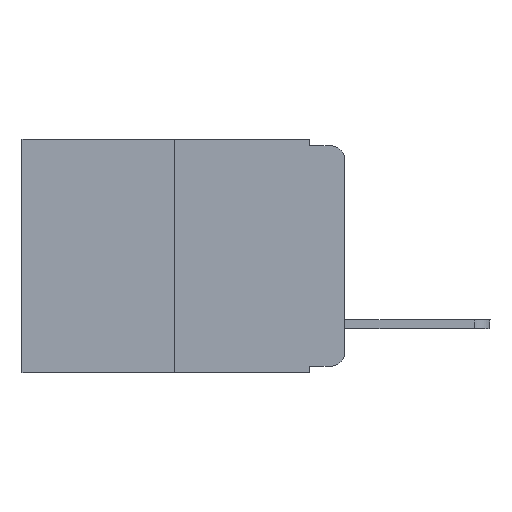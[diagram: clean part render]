
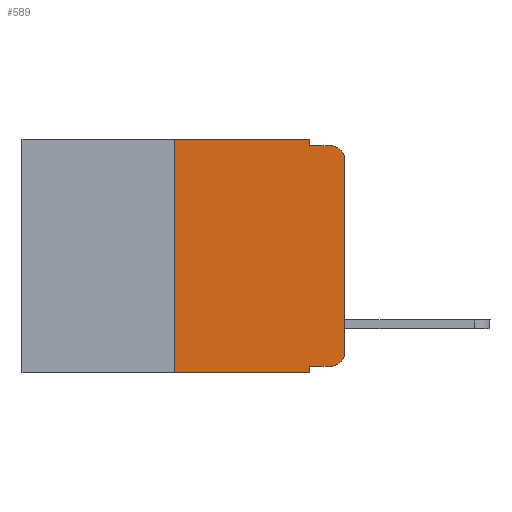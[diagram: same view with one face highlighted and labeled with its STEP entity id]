
A CAD part, left-side view. The second image highlights one B-rep face of the part: STEP entity #589.
In plain terms, the highlighted planar face has unit normal (-1, 0, 0).
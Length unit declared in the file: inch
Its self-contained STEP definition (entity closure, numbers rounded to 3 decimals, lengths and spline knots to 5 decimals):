
#64 = DIRECTION ( 'NONE',  ( 0., -1., 0. ) ) ;
#264 = EDGE_CURVE ( 'NONE', #17933, #17940, #12349, .T. ) ;
#484 = AXIS2_PLACEMENT_3D ( 'NONE', #14368, #19303, #11147 ) ;
#589 = ADVANCED_FACE ( 'NONE', ( #12611 ), #6044, .F. ) ;
#773 = ORIENTED_EDGE ( 'NONE', *, *, #10100, .T. ) ;
#1182 = CARTESIAN_POINT ( 'NONE',  ( 0., 0.051, 0. ) ) ;
#1595 = DIRECTION ( 'NONE',  ( 0., 0., 1. ) ) ;
#1797 = ORIENTED_EDGE ( 'NONE', *, *, #4053, .F. ) ;
#2514 = VERTEX_POINT ( 'NONE', #8550 ) ;
#2700 = CARTESIAN_POINT ( 'NONE',  ( 0., 0., -0.03 ) ) ;
#2999 = CARTESIAN_POINT ( 'NONE',  ( 0., 0., 0. ) ) ;
#3003 = VECTOR ( 'NONE', #1595, 39.37008 ) ;
#3237 = DIRECTION ( 'NONE',  ( 0., 0., -1. ) ) ;
#3683 = ORIENTED_EDGE ( 'NONE', *, *, #20851, .T. ) ;
#3933 = CARTESIAN_POINT ( 'NONE',  ( 0., 0.051, -0.01 ) ) ;
#4053 = EDGE_CURVE ( 'NONE', #6604, #7138, #17782, .T. ) ;
#4544 = CARTESIAN_POINT ( 'NONE',  ( 0., 0.051, 0. ) ) ;
#4572 = CARTESIAN_POINT ( 'NONE',  ( 0., 0.051, -0.333 ) ) ;
#4611 = ORIENTED_EDGE ( 'NONE', *, *, #19996, .F. ) ;
#4743 = ORIENTED_EDGE ( 'NONE', *, *, #8467, .F. ) ;
#4758 = CARTESIAN_POINT ( 'NONE',  ( 0., 0.02, -0.01 ) ) ;
#5147 = ORIENTED_EDGE ( 'NONE', *, *, #264, .T. ) ;
#6044 = PLANE ( 'NONE',  #15640 ) ;
#6058 = DIRECTION ( 'NONE',  ( 0., 0., -1. ) ) ;
#6085 = LINE ( 'NONE', #4572, #15547 ) ;
#6604 = VERTEX_POINT ( 'NONE', #19580 ) ;
#6805 = DIRECTION ( 'NONE',  ( -1., 0., 0. ) ) ;
#7040 = CIRCLE ( 'NONE', #484, 0.02 ) ;
#7138 = VERTEX_POINT ( 'NONE', #3933 ) ;
#7621 = CARTESIAN_POINT ( 'NONE',  ( 0., 0.02, -0.333 ) ) ;
#7890 = CARTESIAN_POINT ( 'NONE',  ( 0., 0.051, -0.01 ) ) ;
#8227 = VERTEX_POINT ( 'NONE', #18062 ) ;
#8467 = EDGE_CURVE ( 'NONE', #8227, #13539, #11939, .T. ) ;
#8550 = CARTESIAN_POINT ( 'NONE',  ( 0., 0., -0.313 ) ) ;
#9002 = ORIENTED_EDGE ( 'NONE', *, *, #15428, .T. ) ;
#9029 = CARTESIAN_POINT ( 'NONE',  ( 0., 0.25, 0. ) ) ;
#9471 = VECTOR ( 'NONE', #12783, 39.37008 ) ;
#9500 = CARTESIAN_POINT ( 'NONE',  ( 0., 0.473, 0. ) ) ;
#9531 = EDGE_CURVE ( 'NONE', #7138, #17940, #14756, .T. ) ;
#9762 = DIRECTION ( 'NONE',  ( 0., -1., 0. ) ) ;
#10100 = EDGE_CURVE ( 'NONE', #15686, #2514, #7040, .T. ) ;
#10711 = VECTOR ( 'NONE', #64, 39.37008 ) ;
#10806 = LINE ( 'NONE', #4544, #18174 ) ;
#11015 = DIRECTION ( 'NONE',  ( 0., -1., 0. ) ) ;
#11147 = DIRECTION ( 'NONE',  ( 0., 0., -1. ) ) ;
#11233 = VECTOR ( 'NONE', #11015, 39.37008 ) ;
#11670 = EDGE_CURVE ( 'NONE', #8227, #17687, #14346, .T. ) ;
#11675 = AXIS2_PLACEMENT_3D ( 'NONE', #14669, #6805, #3237 ) ;
#11805 = ORIENTED_EDGE ( 'NONE', *, *, #9531, .F. ) ;
#11939 = LINE ( 'NONE', #9029, #9471 ) ;
#12317 = DIRECTION ( 'NONE',  ( 0., 0., -1. ) ) ;
#12349 = CIRCLE ( 'NONE', #11675, 0.02 ) ;
#12507 = DIRECTION ( 'NONE',  ( 1., 0., 0. ) ) ;
#12611 = FACE_OUTER_BOUND ( 'NONE', #18656, .T. ) ;
#12783 = DIRECTION ( 'NONE',  ( 0., 0., 1. ) ) ;
#12828 = DIRECTION ( 'NONE',  ( 0., 0., -1. ) ) ;
#13131 = CARTESIAN_POINT ( 'NONE',  ( 0., 0.473, 0. ) ) ;
#13150 = LINE ( 'NONE', #2999, #3003 ) ;
#13481 = VECTOR ( 'NONE', #6058, 39.37008 ) ;
#13539 = VERTEX_POINT ( 'NONE', #15063 ) ;
#13694 = ORIENTED_EDGE ( 'NONE', *, *, #17883, .F. ) ;
#14346 = LINE ( 'NONE', #19167, #11233 ) ;
#14368 = CARTESIAN_POINT ( 'NONE',  ( 0., 0.02, -0.313 ) ) ;
#14669 = CARTESIAN_POINT ( 'NONE',  ( 0., 0.02, -0.03 ) ) ;
#14716 = VERTEX_POINT ( 'NONE', #20277 ) ;
#14756 = LINE ( 'NONE', #7890, #17389 ) ;
#15063 = CARTESIAN_POINT ( 'NONE',  ( 0., 0.25, 0. ) ) ;
#15428 = EDGE_CURVE ( 'NONE', #2514, #17933, #13150, .T. ) ;
#15547 = VECTOR ( 'NONE', #9762, 39.37008 ) ;
#15640 = AXIS2_PLACEMENT_3D ( 'NONE', #9500, #12507, #12828 ) ;
#15686 = VERTEX_POINT ( 'NONE', #7621 ) ;
#16377 = DIRECTION ( 'NONE',  ( 0., -1., 0. ) ) ;
#16940 = CARTESIAN_POINT ( 'NONE',  ( 0., 0.051, -0.343 ) ) ;
#17389 = VECTOR ( 'NONE', #16377, 39.37008 ) ;
#17687 = VERTEX_POINT ( 'NONE', #16940 ) ;
#17759 = LINE ( 'NONE', #13131, #10711 ) ;
#17782 = LINE ( 'NONE', #1182, #13481 ) ;
#17883 = EDGE_CURVE ( 'NONE', #14716, #17687, #10806, .T. ) ;
#17922 = ORIENTED_EDGE ( 'NONE', *, *, #11670, .T. ) ;
#17933 = VERTEX_POINT ( 'NONE', #2700 ) ;
#17940 = VERTEX_POINT ( 'NONE', #4758 ) ;
#18062 = CARTESIAN_POINT ( 'NONE',  ( 0., 0.25, -0.343 ) ) ;
#18174 = VECTOR ( 'NONE', #12317, 39.37008 ) ;
#18656 = EDGE_LOOP ( 'NONE', ( #9002, #5147, #11805, #1797, #4611, #4743, #17922, #13694, #3683, #773 ) ) ;
#19167 = CARTESIAN_POINT ( 'NONE',  ( 0., 0.473, -0.343 ) ) ;
#19303 = DIRECTION ( 'NONE',  ( -1., 0., 0. ) ) ;
#19580 = CARTESIAN_POINT ( 'NONE',  ( 0., 0.051, 0. ) ) ;
#19996 = EDGE_CURVE ( 'NONE', #13539, #6604, #17759, .T. ) ;
#20277 = CARTESIAN_POINT ( 'NONE',  ( 0., 0.051, -0.333 ) ) ;
#20851 = EDGE_CURVE ( 'NONE', #14716, #15686, #6085, .T. ) ;
